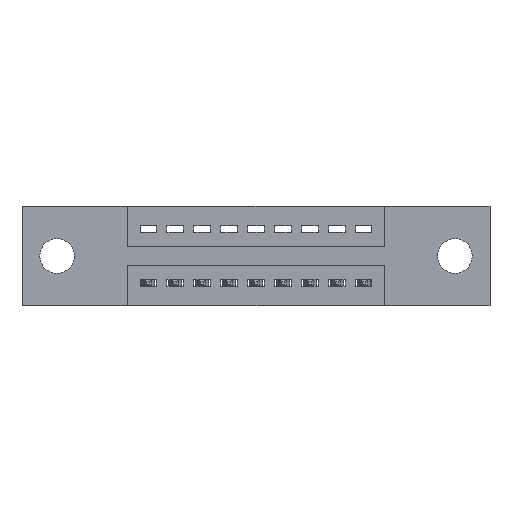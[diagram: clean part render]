
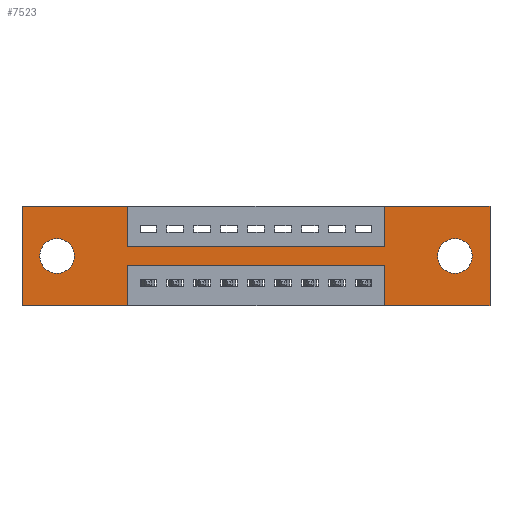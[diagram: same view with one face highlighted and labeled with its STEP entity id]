
A CAD part, front view. The second image highlights one B-rep face of the part: STEP entity #7523.
In plain terms, the highlighted planar face has unit normal (0, -1, 0).
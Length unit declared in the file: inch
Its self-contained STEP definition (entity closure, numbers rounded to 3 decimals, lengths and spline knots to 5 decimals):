
#23 = DIRECTION ( 'NONE',  ( 0., 0., -1. ) ) ;
#59 = LINE ( 'NONE', #10069, #3909 ) ;
#124 = CARTESIAN_POINT ( 'NONE',  ( 0.13, 0., -0.249 ) ) ;
#230 = DIRECTION ( 'NONE',  ( 0., 0., 1. ) ) ;
#247 = DIRECTION ( 'NONE',  ( -1., 0., 0. ) ) ;
#647 = AXIS2_PLACEMENT_3D ( 'NONE', #4035, #10155, #4164 ) ;
#664 = CARTESIAN_POINT ( 'NONE',  ( 0., 0., -0.37 ) ) ;
#715 = VECTOR ( 'NONE', #2421, 39.37008 ) ;
#912 = AXIS2_PLACEMENT_3D ( 'NONE', #1077, #7125, #7199 ) ;
#934 = VERTEX_POINT ( 'NONE', #9751 ) ;
#1005 = VERTEX_POINT ( 'NONE', #10128 ) ;
#1061 = AXIS2_PLACEMENT_3D ( 'NONE', #1080, #10659, #5455 ) ;
#1074 = VECTOR ( 'NONE', #8944, 39.37008 ) ;
#1077 = CARTESIAN_POINT ( 'NONE',  ( 1.605, 0., -0.185 ) ) ;
#1080 = CARTESIAN_POINT ( 'NONE',  ( 0.13, 0., -0.185 ) ) ;
#1136 = CARTESIAN_POINT ( 'NONE',  ( 0., 0., -0.37 ) ) ;
#1156 = CARTESIAN_POINT ( 'NONE',  ( 1.3425, 0., 0. ) ) ;
#1307 = LINE ( 'NONE', #4564, #3756 ) ;
#1324 = EDGE_CURVE ( 'NONE', #2153, #934, #5719, .T. ) ;
#1362 = CIRCLE ( 'NONE', #647, 0.064 ) ;
#1375 = VERTEX_POINT ( 'NONE', #4027 ) ;
#1401 = CARTESIAN_POINT ( 'NONE',  ( 0.3925, 0., 0. ) ) ;
#1730 = CARTESIAN_POINT ( 'NONE',  ( 1.735, 0., 0. ) ) ;
#1779 = CARTESIAN_POINT ( 'NONE',  ( 1.3425, 0., -0.22 ) ) ;
#1792 = VECTOR ( 'NONE', #247, 39.37008 ) ;
#1854 = LINE ( 'NONE', #2350, #6997 ) ;
#1860 = EDGE_LOOP ( 'NONE', ( #3652, #11139 ) ) ;
#1905 = CARTESIAN_POINT ( 'NONE',  ( 0., 0., 0. ) ) ;
#1927 = LINE ( 'NONE', #5154, #8330 ) ;
#1964 = ORIENTED_EDGE ( 'NONE', *, *, #5504, .F. ) ;
#2153 = VERTEX_POINT ( 'NONE', #7832 ) ;
#2162 = DIRECTION ( 'NONE',  ( 0., 0., 1. ) ) ;
#2350 = CARTESIAN_POINT ( 'NONE',  ( 0., 0., 0. ) ) ;
#2421 = DIRECTION ( 'NONE',  ( -1., 0., 0. ) ) ;
#2456 = CARTESIAN_POINT ( 'NONE',  ( 0.3925, 0., -0.22 ) ) ;
#2517 = VERTEX_POINT ( 'NONE', #124 ) ;
#2619 = EDGE_CURVE ( 'NONE', #2670, #2517, #1362, .T. ) ;
#2665 = VECTOR ( 'NONE', #7689, 39.37008 ) ;
#2670 = VERTEX_POINT ( 'NONE', #3386 ) ;
#2683 = EDGE_CURVE ( 'NONE', #9450, #5277, #7873, .T. ) ;
#2797 = VERTEX_POINT ( 'NONE', #3656 ) ;
#2836 = CIRCLE ( 'NONE', #912, 0.064 ) ;
#2920 = VERTEX_POINT ( 'NONE', #8092 ) ;
#3199 = EDGE_LOOP ( 'NONE', ( #10481, #5609, #3482, #8943, #11001, #6580, #3459, #5786, #6139, #7674, #4151, #1964 ) ) ;
#3386 = CARTESIAN_POINT ( 'NONE',  ( 0.13, 0., -0.121 ) ) ;
#3445 = DIRECTION ( 'NONE',  ( 0., 1., 0. ) ) ;
#3459 = ORIENTED_EDGE ( 'NONE', *, *, #8857, .F. ) ;
#3482 = ORIENTED_EDGE ( 'NONE', *, *, #9617, .F. ) ;
#3544 = VECTOR ( 'NONE', #6376, 39.37008 ) ;
#3652 = ORIENTED_EDGE ( 'NONE', *, *, #2619, .T. ) ;
#3656 = CARTESIAN_POINT ( 'NONE',  ( 0., 0., 0. ) ) ;
#3686 = EDGE_CURVE ( 'NONE', #7023, #1005, #10675, .T. ) ;
#3756 = VECTOR ( 'NONE', #230, 39.37008 ) ;
#3765 = VECTOR ( 'NONE', #7231, 39.37008 ) ;
#3808 = EDGE_CURVE ( 'NONE', #10850, #5855, #4598, .T. ) ;
#3830 = EDGE_LOOP ( 'NONE', ( #10706, #9891 ) ) ;
#3909 = VECTOR ( 'NONE', #2162, 39.37008 ) ;
#4027 = CARTESIAN_POINT ( 'NONE',  ( 0.3925, 0., -0.37 ) ) ;
#4035 = CARTESIAN_POINT ( 'NONE',  ( 0.13, 0., -0.185 ) ) ;
#4098 = DIRECTION ( 'NONE',  ( 0., 0., 1. ) ) ;
#4151 = ORIENTED_EDGE ( 'NONE', *, *, #5916, .F. ) ;
#4164 = DIRECTION ( 'NONE',  ( 0., 0., 1. ) ) ;
#4381 = VERTEX_POINT ( 'NONE', #1401 ) ;
#4564 = CARTESIAN_POINT ( 'NONE',  ( 1.3425, 0., -0.37 ) ) ;
#4582 = CARTESIAN_POINT ( 'NONE',  ( 0., 0., -0.37 ) ) ;
#4598 = LINE ( 'NONE', #1905, #10285 ) ;
#5038 = VECTOR ( 'NONE', #4098, 39.37008 ) ;
#5138 = CARTESIAN_POINT ( 'NONE',  ( 0.3925, 0., -0.22 ) ) ;
#5154 = CARTESIAN_POINT ( 'NONE',  ( 0.3925, 0., -0.37 ) ) ;
#5277 = VERTEX_POINT ( 'NONE', #2456 ) ;
#5364 = PLANE ( 'NONE',  #6118 ) ;
#5430 = EDGE_CURVE ( 'NONE', #5277, #1375, #1927, .T. ) ;
#5455 = DIRECTION ( 'NONE',  ( 0., 0., 1. ) ) ;
#5504 = EDGE_CURVE ( 'NONE', #1375, #2920, #9563, .T. ) ;
#5609 = ORIENTED_EDGE ( 'NONE', *, *, #2683, .F. ) ;
#5719 = LINE ( 'NONE', #664, #715 ) ;
#5771 = LINE ( 'NONE', #6344, #3765 ) ;
#5786 = ORIENTED_EDGE ( 'NONE', *, *, #8470, .F. ) ;
#5855 = VERTEX_POINT ( 'NONE', #8230 ) ;
#5916 = EDGE_CURVE ( 'NONE', #2920, #2797, #9937, .T. ) ;
#6023 = DIRECTION ( 'NONE',  ( 0., 0., -1. ) ) ;
#6118 = AXIS2_PLACEMENT_3D ( 'NONE', #1136, #6222, #8992 ) ;
#6139 = ORIENTED_EDGE ( 'NONE', *, *, #8969, .F. ) ;
#6198 = LINE ( 'NONE', #1730, #1074 ) ;
#6222 = DIRECTION ( 'NONE',  ( 0., -1., 0. ) ) ;
#6344 = CARTESIAN_POINT ( 'NONE',  ( 0.3925, 0., 0. ) ) ;
#6376 = DIRECTION ( 'NONE',  ( -1., 0., 0. ) ) ;
#6580 = ORIENTED_EDGE ( 'NONE', *, *, #3808, .F. ) ;
#6997 = VECTOR ( 'NONE', #8503, 39.37008 ) ;
#7023 = VERTEX_POINT ( 'NONE', #9758 ) ;
#7047 = EDGE_CURVE ( 'NONE', #2517, #2670, #10030, .T. ) ;
#7066 = VERTEX_POINT ( 'NONE', #9903 ) ;
#7125 = DIRECTION ( 'NONE',  ( 0., 1., 0. ) ) ;
#7134 = EDGE_CURVE ( 'NONE', #1005, #7023, #2836, .T. ) ;
#7153 = CARTESIAN_POINT ( 'NONE',  ( 0.3925, 0., -0.15 ) ) ;
#7199 = DIRECTION ( 'NONE',  ( 0., 0., -1. ) ) ;
#7231 = DIRECTION ( 'NONE',  ( 0., 0., -1. ) ) ;
#7292 = VERTEX_POINT ( 'NONE', #7153 ) ;
#7346 = EDGE_CURVE ( 'NONE', #5855, #2153, #6198, .T. ) ;
#7523 = ADVANCED_FACE ( 'NONE', ( #10699, #8553, #8409 ), #5364, .T. ) ;
#7545 = AXIS2_PLACEMENT_3D ( 'NONE', #11216, #3445, #6023 ) ;
#7674 = ORIENTED_EDGE ( 'NONE', *, *, #8450, .F. ) ;
#7689 = DIRECTION ( 'NONE',  ( 1., 0., 0. ) ) ;
#7832 = CARTESIAN_POINT ( 'NONE',  ( 1.735, 0., -0.37 ) ) ;
#7873 = LINE ( 'NONE', #5138, #3544 ) ;
#7990 = DIRECTION ( 'NONE',  ( 1., 0., 0. ) ) ;
#8092 = CARTESIAN_POINT ( 'NONE',  ( 0., 0., -0.37 ) ) ;
#8230 = CARTESIAN_POINT ( 'NONE',  ( 1.735, 0., 0. ) ) ;
#8330 = VECTOR ( 'NONE', #23, 39.37008 ) ;
#8332 = CARTESIAN_POINT ( 'NONE',  ( 0., 0., 0. ) ) ;
#8409 = FACE_OUTER_BOUND ( 'NONE', #3199, .T. ) ;
#8450 = EDGE_CURVE ( 'NONE', #2797, #4381, #1854, .T. ) ;
#8470 = EDGE_CURVE ( 'NONE', #7292, #7066, #9486, .T. ) ;
#8503 = DIRECTION ( 'NONE',  ( 1., 0., 0. ) ) ;
#8553 = FACE_BOUND ( 'NONE', #1860, .T. ) ;
#8584 = CARTESIAN_POINT ( 'NONE',  ( 0.3925, 0., -0.15 ) ) ;
#8857 = EDGE_CURVE ( 'NONE', #7066, #10850, #59, .T. ) ;
#8943 = ORIENTED_EDGE ( 'NONE', *, *, #1324, .F. ) ;
#8944 = DIRECTION ( 'NONE',  ( 0., 0., -1. ) ) ;
#8969 = EDGE_CURVE ( 'NONE', #4381, #7292, #5771, .T. ) ;
#8992 = DIRECTION ( 'NONE',  ( 0., 0., -1. ) ) ;
#9450 = VERTEX_POINT ( 'NONE', #1779 ) ;
#9486 = LINE ( 'NONE', #8584, #2665 ) ;
#9563 = LINE ( 'NONE', #4582, #1792 ) ;
#9617 = EDGE_CURVE ( 'NONE', #934, #9450, #1307, .T. ) ;
#9751 = CARTESIAN_POINT ( 'NONE',  ( 1.3425, 0., -0.37 ) ) ;
#9758 = CARTESIAN_POINT ( 'NONE',  ( 1.605, 0., -0.249 ) ) ;
#9891 = ORIENTED_EDGE ( 'NONE', *, *, #3686, .T. ) ;
#9903 = CARTESIAN_POINT ( 'NONE',  ( 1.3425, 0., -0.15 ) ) ;
#9937 = LINE ( 'NONE', #8332, #5038 ) ;
#10030 = CIRCLE ( 'NONE', #1061, 0.064 ) ;
#10069 = CARTESIAN_POINT ( 'NONE',  ( 1.3425, 0., 0. ) ) ;
#10128 = CARTESIAN_POINT ( 'NONE',  ( 1.605, 0., -0.121 ) ) ;
#10155 = DIRECTION ( 'NONE',  ( 0., 1., 0. ) ) ;
#10285 = VECTOR ( 'NONE', #7990, 39.37008 ) ;
#10481 = ORIENTED_EDGE ( 'NONE', *, *, #5430, .F. ) ;
#10659 = DIRECTION ( 'NONE',  ( 0., 1., 0. ) ) ;
#10675 = CIRCLE ( 'NONE', #7545, 0.064 ) ;
#10699 = FACE_BOUND ( 'NONE', #3830, .T. ) ;
#10706 = ORIENTED_EDGE ( 'NONE', *, *, #7134, .T. ) ;
#10850 = VERTEX_POINT ( 'NONE', #1156 ) ;
#11001 = ORIENTED_EDGE ( 'NONE', *, *, #7346, .F. ) ;
#11139 = ORIENTED_EDGE ( 'NONE', *, *, #7047, .T. ) ;
#11216 = CARTESIAN_POINT ( 'NONE',  ( 1.605, 0., -0.185 ) ) ;
